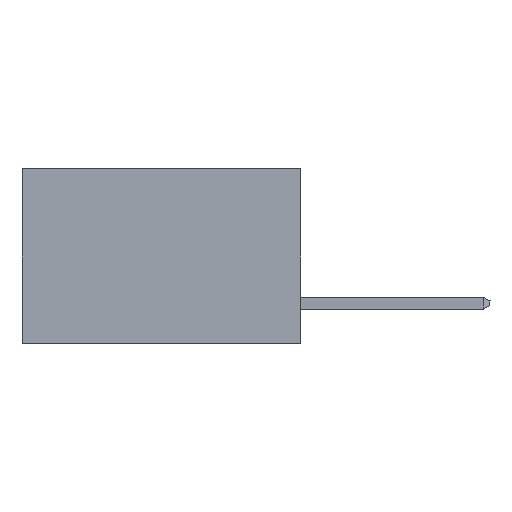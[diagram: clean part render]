
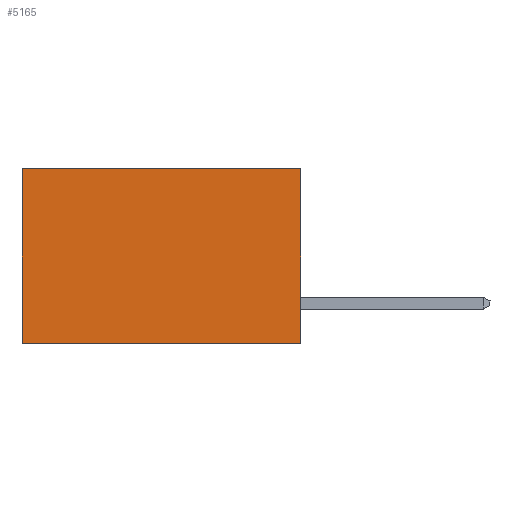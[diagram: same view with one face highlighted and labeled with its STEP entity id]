
A CAD part, left-side view. The second image highlights one B-rep face of the part: STEP entity #5165.
In plain terms, the highlighted planar face has unit normal (-1, 0, 0).
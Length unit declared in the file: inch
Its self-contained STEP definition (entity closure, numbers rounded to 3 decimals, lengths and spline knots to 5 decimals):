
#237 = LINE ( 'NONE', #10011, #10529 ) ;
#823 = CARTESIAN_POINT ( 'NONE',  ( 0.277, 0., 0. ) ) ;
#1010 = DIRECTION ( 'NONE',  ( 0., 1., 0. ) ) ;
#1512 = ORIENTED_EDGE ( 'NONE', *, *, #2673, .F. ) ;
#2137 = EDGE_CURVE ( 'NONE', #7313, #4355, #237, .T. ) ;
#2179 = DIRECTION ( 'NONE',  ( 0., 0., -1. ) ) ;
#2250 = DIRECTION ( 'NONE',  ( 0., 1., 0. ) ) ;
#2296 = DIRECTION ( 'NONE',  ( 1., 0., 0. ) ) ;
#2366 = CARTESIAN_POINT ( 'NONE',  ( 0.277, 0., -0.37 ) ) ;
#2369 = PLANE ( 'NONE',  #4398 ) ;
#2558 = ORIENTED_EDGE ( 'NONE', *, *, #13694, .T. ) ;
#2673 = EDGE_CURVE ( 'NONE', #9876, #7313, #12656, .T. ) ;
#3825 = ORIENTED_EDGE ( 'NONE', *, *, #14134, .T. ) ;
#4355 = VERTEX_POINT ( 'NONE', #14153 ) ;
#4398 = AXIS2_PLACEMENT_3D ( 'NONE', #2366, #2296, #2179 ) ;
#5165 = ADVANCED_FACE ( 'NONE', ( #10410 ), #2369, .F. ) ;
#5596 = DIRECTION ( 'NONE',  ( 0., 0., -1. ) ) ;
#5782 = VERTEX_POINT ( 'NONE', #17894 ) ;
#6348 = ORIENTED_EDGE ( 'NONE', *, *, #2137, .F. ) ;
#7313 = VERTEX_POINT ( 'NONE', #15653 ) ;
#8295 = EDGE_LOOP ( 'NONE', ( #2558, #6348, #1512, #3825 ) ) ;
#9002 = VECTOR ( 'NONE', #12070, 39.37008 ) ;
#9785 = VECTOR ( 'NONE', #2250, 39.37008 ) ;
#9805 = LINE ( 'NONE', #18052, #16364 ) ;
#9876 = VERTEX_POINT ( 'NONE', #12343 ) ;
#10011 = CARTESIAN_POINT ( 'NONE',  ( 0.277, 0., -0.37 ) ) ;
#10410 = FACE_OUTER_BOUND ( 'NONE', #8295, .T. ) ;
#10529 = VECTOR ( 'NONE', #1010, 39.37008 ) ;
#12070 = DIRECTION ( 'NONE',  ( 0., 0., -1. ) ) ;
#12233 = CARTESIAN_POINT ( 'NONE',  ( 0.277, 0., -0.37 ) ) ;
#12343 = CARTESIAN_POINT ( 'NONE',  ( 0.277, 0., 0. ) ) ;
#12656 = LINE ( 'NONE', #12233, #9002 ) ;
#12997 = LINE ( 'NONE', #823, #9785 ) ;
#13694 = EDGE_CURVE ( 'NONE', #5782, #4355, #9805, .T. ) ;
#14134 = EDGE_CURVE ( 'NONE', #9876, #5782, #12997, .T. ) ;
#14153 = CARTESIAN_POINT ( 'NONE',  ( 0.277, 0.59, -0.37 ) ) ;
#15653 = CARTESIAN_POINT ( 'NONE',  ( 0.277, 0., -0.37 ) ) ;
#16364 = VECTOR ( 'NONE', #5596, 39.37008 ) ;
#17894 = CARTESIAN_POINT ( 'NONE',  ( 0.277, 0.59, 0. ) ) ;
#18052 = CARTESIAN_POINT ( 'NONE',  ( 0.277, 0.59, -0.37 ) ) ;
